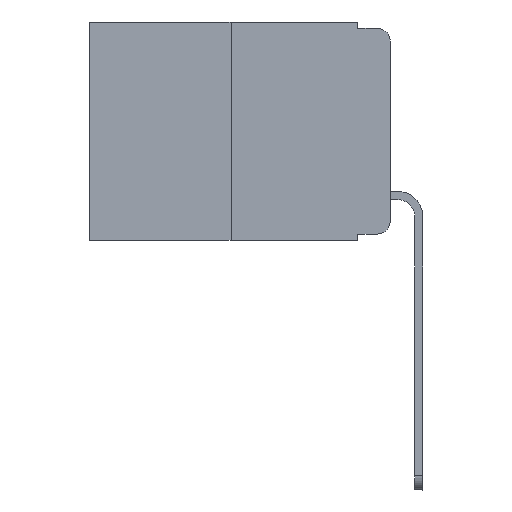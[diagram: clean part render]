
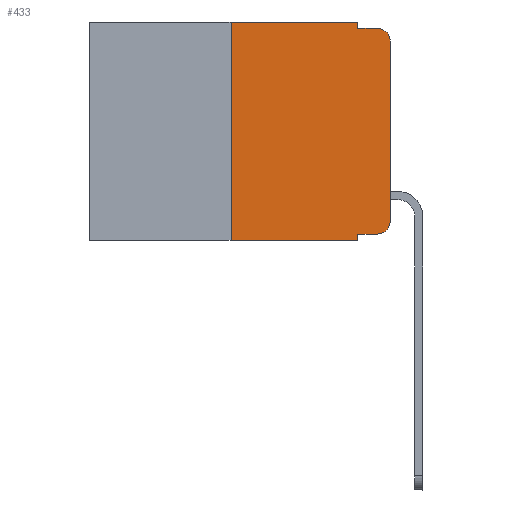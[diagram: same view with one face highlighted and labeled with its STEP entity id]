
A CAD part, left-side view. The second image highlights one B-rep face of the part: STEP entity #433.
In plain terms, the highlighted planar face has unit normal (-1, 0, 0).
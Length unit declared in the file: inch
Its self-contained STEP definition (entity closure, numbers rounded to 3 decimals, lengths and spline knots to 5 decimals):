
#237 = CARTESIAN_POINT ( 'NONE',  ( 0., 0.051, 0. ) ) ;
#383 = ORIENTED_EDGE ( 'NONE', *, *, #16465, .F. ) ;
#433 = ADVANCED_FACE ( 'NONE', ( #6435 ), #9040, .F. ) ;
#545 = CARTESIAN_POINT ( 'NONE',  ( 0., 0.051, -0.343 ) ) ;
#561 = LINE ( 'NONE', #16938, #16160 ) ;
#619 = EDGE_CURVE ( 'NONE', #5817, #5295, #7801, .T. ) ;
#1208 = DIRECTION ( 'NONE',  ( 0., 0., -1. ) ) ;
#1424 = CARTESIAN_POINT ( 'NONE',  ( 0., 0.25, -0.343 ) ) ;
#2103 = DIRECTION ( 'NONE',  ( 1., 0., 0. ) ) ;
#2489 = DIRECTION ( 'NONE',  ( 0., 0., -1. ) ) ;
#2501 = ORIENTED_EDGE ( 'NONE', *, *, #16879, .T. ) ;
#2527 = LINE ( 'NONE', #9542, #16758 ) ;
#2737 = CARTESIAN_POINT ( 'NONE',  ( 0., 0.02, -0.03 ) ) ;
#2956 = VERTEX_POINT ( 'NONE', #12943 ) ;
#3175 = DIRECTION ( 'NONE',  ( 0., -1., 0. ) ) ;
#3362 = LINE ( 'NONE', #14255, #10428 ) ;
#3778 = CARTESIAN_POINT ( 'NONE',  ( 0., 0.051, -0.333 ) ) ;
#3905 = CARTESIAN_POINT ( 'NONE',  ( 0., 0., -0.03 ) ) ;
#5098 = DIRECTION ( 'NONE',  ( 0., 0., -1. ) ) ;
#5245 = DIRECTION ( 'NONE',  ( 0., -1., 0. ) ) ;
#5295 = VERTEX_POINT ( 'NONE', #6691 ) ;
#5450 = DIRECTION ( 'NONE',  ( -1., 0., 0. ) ) ;
#5655 = EDGE_CURVE ( 'NONE', #5817, #8869, #2527, .T. ) ;
#5817 = VERTEX_POINT ( 'NONE', #1424 ) ;
#5865 = VECTOR ( 'NONE', #5098, 39.37008 ) ;
#5872 = AXIS2_PLACEMENT_3D ( 'NONE', #14453, #2103, #7791 ) ;
#6028 = ORIENTED_EDGE ( 'NONE', *, *, #11928, .F. ) ;
#6435 = FACE_OUTER_BOUND ( 'NONE', #7614, .T. ) ;
#6469 = LINE ( 'NONE', #16099, #11304 ) ;
#6617 = CARTESIAN_POINT ( 'NONE',  ( 0., 0.051, 0. ) ) ;
#6691 = CARTESIAN_POINT ( 'NONE',  ( 0., 0.25, 0. ) ) ;
#7008 = CIRCLE ( 'NONE', #14489, 0.02 ) ;
#7020 = AXIS2_PLACEMENT_3D ( 'NONE', #17607, #13294, #2489 ) ;
#7614 = EDGE_LOOP ( 'NONE', ( #2501, #17781, #11597, #383, #7762, #11810, #15657, #6028, #8586, #7760 ) ) ;
#7760 = ORIENTED_EDGE ( 'NONE', *, *, #12885, .T. ) ;
#7762 = ORIENTED_EDGE ( 'NONE', *, *, #8680, .F. ) ;
#7790 = LINE ( 'NONE', #6617, #5865 ) ;
#7791 = DIRECTION ( 'NONE',  ( 0., 0., -1. ) ) ;
#7801 = LINE ( 'NONE', #13380, #11623 ) ;
#8271 = LINE ( 'NONE', #3778, #15985 ) ;
#8335 = CARTESIAN_POINT ( 'NONE',  ( 0., 0., -0.313 ) ) ;
#8586 = ORIENTED_EDGE ( 'NONE', *, *, #14366, .T. ) ;
#8661 = DIRECTION ( 'NONE',  ( 0., -1., 0. ) ) ;
#8680 = EDGE_CURVE ( 'NONE', #5295, #10879, #561, .T. ) ;
#8869 = VERTEX_POINT ( 'NONE', #545 ) ;
#9040 = PLANE ( 'NONE',  #5872 ) ;
#9407 = LINE ( 'NONE', #14894, #17651 ) ;
#9542 = CARTESIAN_POINT ( 'NONE',  ( 0., 0.473, -0.343 ) ) ;
#9650 = VERTEX_POINT ( 'NONE', #12730 ) ;
#9868 = VERTEX_POINT ( 'NONE', #3905 ) ;
#10428 = VECTOR ( 'NONE', #8661, 39.37008 ) ;
#10695 = DIRECTION ( 'NONE',  ( 0., 0., -1. ) ) ;
#10879 = VERTEX_POINT ( 'NONE', #237 ) ;
#11304 = VECTOR ( 'NONE', #10695, 39.37008 ) ;
#11441 = VERTEX_POINT ( 'NONE', #11982 ) ;
#11597 = ORIENTED_EDGE ( 'NONE', *, *, #14874, .F. ) ;
#11623 = VECTOR ( 'NONE', #16495, 39.37008 ) ;
#11810 = ORIENTED_EDGE ( 'NONE', *, *, #619, .F. ) ;
#11928 = EDGE_CURVE ( 'NONE', #9650, #8869, #6469, .T. ) ;
#11982 = CARTESIAN_POINT ( 'NONE',  ( 0., 0.02, -0.01 ) ) ;
#12208 = DIRECTION ( 'NONE',  ( 0., 0., 1. ) ) ;
#12481 = EDGE_CURVE ( 'NONE', #9868, #11441, #7008, .T. ) ;
#12730 = CARTESIAN_POINT ( 'NONE',  ( 0., 0.051, -0.333 ) ) ;
#12885 = EDGE_CURVE ( 'NONE', #2956, #16122, #16796, .T. ) ;
#12943 = CARTESIAN_POINT ( 'NONE',  ( 0., 0.02, -0.333 ) ) ;
#13294 = DIRECTION ( 'NONE',  ( -1., 0., 0. ) ) ;
#13380 = CARTESIAN_POINT ( 'NONE',  ( 0., 0.25, 0. ) ) ;
#14255 = CARTESIAN_POINT ( 'NONE',  ( 0., 0.051, -0.01 ) ) ;
#14366 = EDGE_CURVE ( 'NONE', #9650, #2956, #8271, .T. ) ;
#14453 = CARTESIAN_POINT ( 'NONE',  ( 0., 0.473, 0. ) ) ;
#14459 = VERTEX_POINT ( 'NONE', #15554 ) ;
#14489 = AXIS2_PLACEMENT_3D ( 'NONE', #2737, #5450, #1208 ) ;
#14874 = EDGE_CURVE ( 'NONE', #14459, #11441, #3362, .T. ) ;
#14894 = CARTESIAN_POINT ( 'NONE',  ( 0., 0., 0. ) ) ;
#15554 = CARTESIAN_POINT ( 'NONE',  ( 0., 0.051, -0.01 ) ) ;
#15657 = ORIENTED_EDGE ( 'NONE', *, *, #5655, .T. ) ;
#15985 = VECTOR ( 'NONE', #17717, 39.37008 ) ;
#16099 = CARTESIAN_POINT ( 'NONE',  ( 0., 0.051, 0. ) ) ;
#16122 = VERTEX_POINT ( 'NONE', #8335 ) ;
#16160 = VECTOR ( 'NONE', #3175, 39.37008 ) ;
#16465 = EDGE_CURVE ( 'NONE', #10879, #14459, #7790, .T. ) ;
#16495 = DIRECTION ( 'NONE',  ( 0., 0., 1. ) ) ;
#16758 = VECTOR ( 'NONE', #5245, 39.37008 ) ;
#16796 = CIRCLE ( 'NONE', #7020, 0.02 ) ;
#16879 = EDGE_CURVE ( 'NONE', #16122, #9868, #9407, .T. ) ;
#16938 = CARTESIAN_POINT ( 'NONE',  ( 0., 0.473, 0. ) ) ;
#17607 = CARTESIAN_POINT ( 'NONE',  ( 0., 0.02, -0.313 ) ) ;
#17651 = VECTOR ( 'NONE', #12208, 39.37008 ) ;
#17717 = DIRECTION ( 'NONE',  ( 0., -1., 0. ) ) ;
#17781 = ORIENTED_EDGE ( 'NONE', *, *, #12481, .T. ) ;
